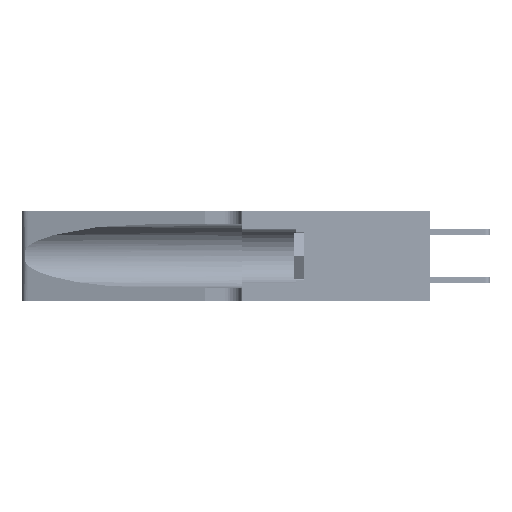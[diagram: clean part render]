
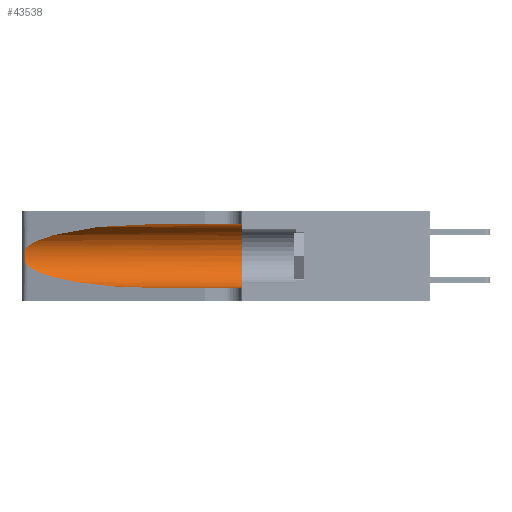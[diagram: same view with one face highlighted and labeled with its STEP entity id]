
A CAD part, left-side view. The second image highlights one B-rep face of the part: STEP entity #43538.
In plain terms, the highlighted cylindrical face has radius 3.308 mm (diameter 6.617 mm), a partial arc.
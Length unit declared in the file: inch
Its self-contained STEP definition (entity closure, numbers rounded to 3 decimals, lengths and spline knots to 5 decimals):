
#1049 = FACE_OUTER_BOUND ( 'NONE', #38258, .T. ) ;
#1362 = CARTESIAN_POINT ( 'NONE',  ( 0.25555, 1.22994, 0.2215 ) ) ;
#1520 = CARTESIAN_POINT ( 'NONE',  ( 0.25487, 1.22718, 0.22369 ) ) ;
#1789 = ORIENTED_EDGE ( 'NONE', *, *, #41856, .F. ) ;
#2274 = CARTESIAN_POINT ( 'NONE',  ( 0.25787, 1.23484, 0.2124 ) ) ;
#2289 = B_SPLINE_CURVE_WITH_KNOTS ( 'NONE', 3,
 ( #1520, #1362, #28933, #2274, #29386, #15728, #26062, #14011, #8644, #23621, #31467, #43469, #38551, #38655 ),
 .UNSPECIFIED., .F., .F.,
 ( 4, 2, 2, 2, 2, 2, 4 ),
 ( 0., 0.00027, 0.00053, 0.00107, 0.0016, 0.00187, 0.00214 ),
 .UNSPECIFIED. ) ;
#2571 = EDGE_CURVE ( 'NONE', #36140, #42321, #40386, .T. ) ;
#2831 = CARTESIAN_POINT ( 'NONE',  ( 0.1305, 0.35, 0.05475 ) ) ;
#3323 = VERTEX_POINT ( 'NONE', #33202 ) ;
#3722 = CYLINDRICAL_SURFACE ( 'NONE', #38250, 0.13025 ) ;
#5631 = CARTESIAN_POINT ( 'NONE',  ( 0.2373, 1.15595, 0.28018 ) ) ;
#5639 = VERTEX_POINT ( 'NONE', #7547 ) ;
#7547 = CARTESIAN_POINT ( 'NONE',  ( 0.25487, 1.22718, 0.22369 ) ) ;
#8644 = CARTESIAN_POINT ( 'NONE',  ( 0.26017, 1.23833, 0.17102 ) ) ;
#8949 = DIRECTION ( 'NONE',  ( 0., -1., 0. ) ) ;
#10137 = ORIENTED_EDGE ( 'NONE', *, *, #2571, .T. ) ;
#10448 =( BOUNDED_CURVE ( )  B_SPLINE_CURVE ( 3, ( #35391, #35996, #18685, #25710 ),
 .UNSPECIFIED., .F., .F. ) 
 B_SPLINE_CURVE_WITH_KNOTS ( ( 4, 4 ),
 ( 3.44316, 4.71239 ),
 .UNSPECIFIED. ) 
 CURVE ( )  GEOMETRIC_REPRESENTATION_ITEM ( )  RATIONAL_B_SPLINE_CURVE ( ( 1., 0.87, 0.87, 1. ) ) 
 REPRESENTATION_ITEM ( '' )  );
#10543 = CARTESIAN_POINT ( 'NONE',  ( 0.25487, 1.22718, 0.14631 ) ) ;
#10737 = ORIENTED_EDGE ( 'NONE', *, *, #13682, .T. ) ;
#10826 = CIRCLE ( 'NONE', #26242, 0.13025 ) ;
#13443 = DIRECTION ( 'NONE',  ( 0., 1., 0. ) ) ;
#13682 = EDGE_CURVE ( 'NONE', #15932, #5639, #34061, .T. ) ;
#14011 = CARTESIAN_POINT ( 'NONE',  ( 0.26075, 1.23896, 0.178 ) ) ;
#14386 = EDGE_CURVE ( 'NONE', #5639, #42543, #2289, .T. ) ;
#15728 = CARTESIAN_POINT ( 'NONE',  ( 0.26018, 1.23835, 0.19895 ) ) ;
#15932 = VERTEX_POINT ( 'NONE', #31356 ) ;
#16200 = DIRECTION ( 'NONE',  ( 0., 0., -1. ) ) ;
#16539 = CARTESIAN_POINT ( 'NONE',  ( 0.1305, 1.61858, 0.31525 ) ) ;
#18685 = CARTESIAN_POINT ( 'NONE',  ( 0.18966, 0.96281, 0.05475 ) ) ;
#20540 = DIRECTION ( 'NONE',  ( 0., 0., 1. ) ) ;
#23621 = CARTESIAN_POINT ( 'NONE',  ( 0.25856, 1.23593, 0.16098 ) ) ;
#24323 = VECTOR ( 'NONE', #8949, 39.37008 ) ;
#25710 = CARTESIAN_POINT ( 'NONE',  ( 0.1305, 0.72297, 0.05475 ) ) ;
#25719 = CARTESIAN_POINT ( 'NONE',  ( 0.1305, 0.72297, 0.31525 ) ) ;
#26062 = CARTESIAN_POINT ( 'NONE',  ( 0.26075, 1.23896, 0.19203 ) ) ;
#26242 = AXIS2_PLACEMENT_3D ( 'NONE', #33956, #13443, #20540 ) ;
#26799 = LINE ( 'NONE', #16539, #41746 ) ;
#28933 = CARTESIAN_POINT ( 'NONE',  ( 0.25639, 1.23184, 0.21858 ) ) ;
#29042 = CARTESIAN_POINT ( 'NONE',  ( 0.18966, 0.96281, 0.31525 ) ) ;
#29187 = CARTESIAN_POINT ( 'NONE',  ( 0.25487, 1.22718, 0.22369 ) ) ;
#29386 = CARTESIAN_POINT ( 'NONE',  ( 0.25854, 1.2359, 0.20912 ) ) ;
#30471 = CARTESIAN_POINT ( 'NONE',  ( 0.1305, 0.72297, 0.05475 ) ) ;
#30595 = DIRECTION ( 'NONE',  ( 0., -1., 0. ) ) ;
#31138 = ORIENTED_EDGE ( 'NONE', *, *, #35790, .T. ) ;
#31356 = CARTESIAN_POINT ( 'NONE',  ( 0.1305, 0.72297, 0.31525 ) ) ;
#31467 = CARTESIAN_POINT ( 'NONE',  ( 0.25789, 1.23486, 0.15765 ) ) ;
#32431 = CARTESIAN_POINT ( 'NONE',  ( 0.1305, 1.61858, 0.05475 ) ) ;
#32937 = DIRECTION ( 'NONE',  ( 0., -1., 0. ) ) ;
#33202 = CARTESIAN_POINT ( 'NONE',  ( 0.1305, 0.35, 0.31525 ) ) ;
#33956 = CARTESIAN_POINT ( 'NONE',  ( 0.1305, 0.35, 0.185 ) ) ;
#34061 =( BOUNDED_CURVE ( )  B_SPLINE_CURVE ( 3, ( #25719, #29042, #5631, #29187 ),
 .UNSPECIFIED., .F., .T. ) 
 B_SPLINE_CURVE_WITH_KNOTS ( ( 4, 4 ),
 ( 1.5708, 2.84003 ),
 .UNSPECIFIED. ) 
 CURVE ( )  GEOMETRIC_REPRESENTATION_ITEM ( )  RATIONAL_B_SPLINE_CURVE ( ( 1., 0.87, 0.87, 1. ) ) 
 REPRESENTATION_ITEM ( '' )  );
#34256 = EDGE_CURVE ( 'NONE', #15932, #3323, #26799, .T. ) ;
#35391 = CARTESIAN_POINT ( 'NONE',  ( 0.25487, 1.22718, 0.14631 ) ) ;
#35790 = EDGE_CURVE ( 'NONE', #42543, #36140, #10448, .T. ) ;
#35996 = CARTESIAN_POINT ( 'NONE',  ( 0.2373, 1.15595, 0.08982 ) ) ;
#36140 = VERTEX_POINT ( 'NONE', #30471 ) ;
#38250 = AXIS2_PLACEMENT_3D ( 'NONE', #43443, #32937, #16200 ) ;
#38253 = ORIENTED_EDGE ( 'NONE', *, *, #14386, .T. ) ;
#38258 = EDGE_LOOP ( 'NONE', ( #10737, #38253, #31138, #10137, #1789, #39773 ) ) ;
#38551 = CARTESIAN_POINT ( 'NONE',  ( 0.25555, 1.22993, 0.14849 ) ) ;
#38655 = CARTESIAN_POINT ( 'NONE',  ( 0.25487, 1.22718, 0.14631 ) ) ;
#39773 = ORIENTED_EDGE ( 'NONE', *, *, #34256, .F. ) ;
#40386 = LINE ( 'NONE', #32431, #24323 ) ;
#41746 = VECTOR ( 'NONE', #30595, 39.37008 ) ;
#41856 = EDGE_CURVE ( 'NONE', #3323, #42321, #10826, .T. ) ;
#42321 = VERTEX_POINT ( 'NONE', #2831 ) ;
#42543 = VERTEX_POINT ( 'NONE', #10543 ) ;
#43443 = CARTESIAN_POINT ( 'NONE',  ( 0.1305, 1.61858, 0.185 ) ) ;
#43469 = CARTESIAN_POINT ( 'NONE',  ( 0.25639, 1.23186, 0.15144 ) ) ;
#43538 = ADVANCED_FACE ( 'NONE', ( #1049 ), #3722, .F. ) ;
